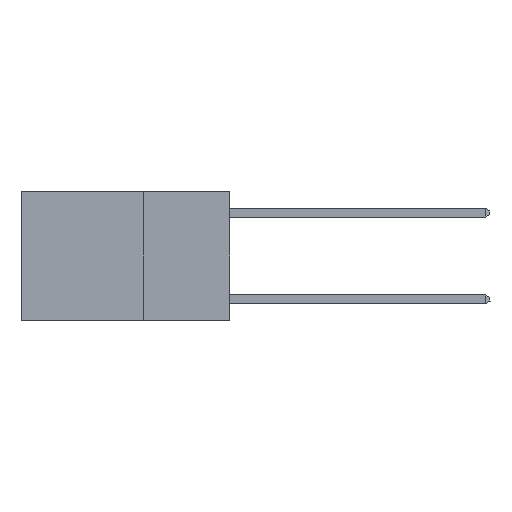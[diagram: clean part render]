
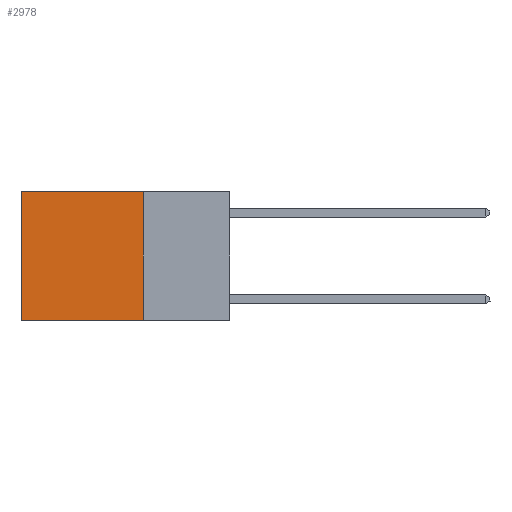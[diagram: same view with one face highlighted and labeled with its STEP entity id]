
A CAD part, left-side view. The second image highlights one B-rep face of the part: STEP entity #2978.
In plain terms, the highlighted planar face has unit normal (-1, 0, 0).
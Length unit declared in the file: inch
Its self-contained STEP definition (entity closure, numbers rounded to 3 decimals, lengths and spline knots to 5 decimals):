
#101 = CARTESIAN_POINT ( 'NONE',  ( 0.2625, 0.6, 0. ) ) ;
#416 = VERTEX_POINT ( 'NONE', #21078 ) ;
#1476 = ORIENTED_EDGE ( 'NONE', *, *, #12480, .F. ) ;
#1519 = DIRECTION ( 'NONE',  ( 0., 0., -1. ) ) ;
#1574 = DIRECTION ( 'NONE',  ( 0., 0., -1. ) ) ;
#2209 = ORIENTED_EDGE ( 'NONE', *, *, #5771, .F. ) ;
#2978 = ADVANCED_FACE ( 'NONE', ( #19710 ), #27390, .F. ) ;
#3013 = CARTESIAN_POINT ( 'NONE',  ( 0.2625, 0.25, 0. ) ) ;
#4016 = VERTEX_POINT ( 'NONE', #101 ) ;
#5110 = ORIENTED_EDGE ( 'NONE', *, *, #13705, .T. ) ;
#5771 = EDGE_CURVE ( 'NONE', #8663, #26402, #25755, .T. ) ;
#6385 = VECTOR ( 'NONE', #1519, 39.37008 ) ;
#7028 = LINE ( 'NONE', #10836, #17865 ) ;
#8663 = VERTEX_POINT ( 'NONE', #22191 ) ;
#9743 = EDGE_LOOP ( 'NONE', ( #23273, #1476, #2209, #5110 ) ) ;
#10014 = AXIS2_PLACEMENT_3D ( 'NONE', #19087, #14996, #1574 ) ;
#10401 = VECTOR ( 'NONE', #18402, 39.37008 ) ;
#10836 = CARTESIAN_POINT ( 'NONE',  ( 0.2625, 0.25, -0.37 ) ) ;
#10860 = EDGE_CURVE ( 'NONE', #4016, #416, #12397, .T. ) ;
#12397 = LINE ( 'NONE', #21137, #6385 ) ;
#12480 = EDGE_CURVE ( 'NONE', #26402, #416, #7028, .T. ) ;
#12974 = DIRECTION ( 'NONE',  ( 0., 1., 0. ) ) ;
#13705 = EDGE_CURVE ( 'NONE', #8663, #4016, #22059, .T. ) ;
#14505 = CARTESIAN_POINT ( 'NONE',  ( 0.2625, 0.25, 0. ) ) ;
#14996 = DIRECTION ( 'NONE',  ( 1., 0., 0. ) ) ;
#16584 = DIRECTION ( 'NONE',  ( 0., 1., 0. ) ) ;
#17865 = VECTOR ( 'NONE', #12974, 39.37008 ) ;
#18111 = CARTESIAN_POINT ( 'NONE',  ( 0.2625, 0.25, -0.37 ) ) ;
#18402 = DIRECTION ( 'NONE',  ( 0., 0., -1. ) ) ;
#19087 = CARTESIAN_POINT ( 'NONE',  ( 0.2625, 0.25, 0. ) ) ;
#19710 = FACE_OUTER_BOUND ( 'NONE', #9743, .T. ) ;
#21078 = CARTESIAN_POINT ( 'NONE',  ( 0.2625, 0.6, -0.37 ) ) ;
#21137 = CARTESIAN_POINT ( 'NONE',  ( 0.2625, 0.6, 0. ) ) ;
#22059 = LINE ( 'NONE', #14505, #27506 ) ;
#22191 = CARTESIAN_POINT ( 'NONE',  ( 0.2625, 0.25, 0. ) ) ;
#23273 = ORIENTED_EDGE ( 'NONE', *, *, #10860, .T. ) ;
#25755 = LINE ( 'NONE', #3013, #10401 ) ;
#26402 = VERTEX_POINT ( 'NONE', #18111 ) ;
#27390 = PLANE ( 'NONE',  #10014 ) ;
#27506 = VECTOR ( 'NONE', #16584, 39.37008 ) ;
